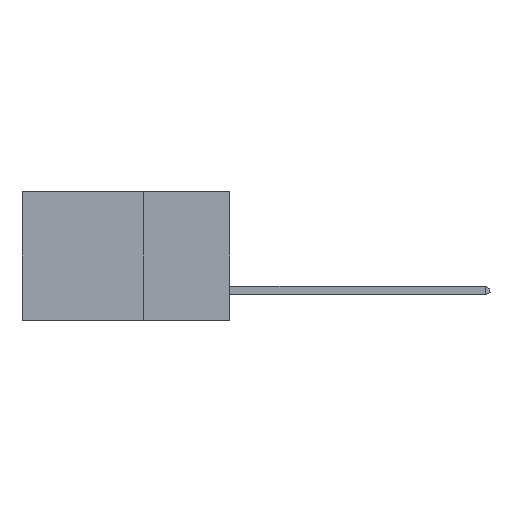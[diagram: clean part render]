
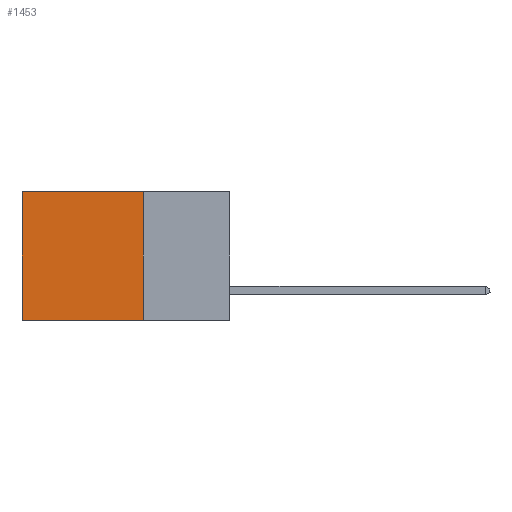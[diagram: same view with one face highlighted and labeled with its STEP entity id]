
A CAD part, left-side view. The second image highlights one B-rep face of the part: STEP entity #1453.
In plain terms, the highlighted planar face has unit normal (-1, 0, 0).
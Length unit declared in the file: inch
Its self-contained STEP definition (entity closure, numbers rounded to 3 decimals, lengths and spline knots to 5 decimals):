
#591 = VERTEX_POINT ( 'NONE', #19879 ) ;
#1293 = EDGE_LOOP ( 'NONE', ( #11337, #5749, #17650, #3230 ) ) ;
#1453 = ADVANCED_FACE ( 'NONE', ( #4125 ), #7468, .F. ) ;
#1702 = VECTOR ( 'NONE', #20775, 39.37008 ) ;
#2573 = DIRECTION ( 'NONE',  ( 0., 0., -1. ) ) ;
#2679 = CARTESIAN_POINT ( 'NONE',  ( 0.298, 0.6, 0. ) ) ;
#2798 = VECTOR ( 'NONE', #12227, 39.37008 ) ;
#3116 = CARTESIAN_POINT ( 'NONE',  ( 0.298, 0.25, -0.37 ) ) ;
#3230 = ORIENTED_EDGE ( 'NONE', *, *, #4395, .T. ) ;
#3769 = VERTEX_POINT ( 'NONE', #10613 ) ;
#4125 = FACE_OUTER_BOUND ( 'NONE', #1293, .T. ) ;
#4395 = EDGE_CURVE ( 'NONE', #3769, #591, #15009, .T. ) ;
#5201 = EDGE_CURVE ( 'NONE', #591, #13915, #13582, .T. ) ;
#5749 = ORIENTED_EDGE ( 'NONE', *, *, #13955, .F. ) ;
#7468 = PLANE ( 'NONE',  #7604 ) ;
#7575 = VERTEX_POINT ( 'NONE', #3116 ) ;
#7604 = AXIS2_PLACEMENT_3D ( 'NONE', #18909, #10744, #2573 ) ;
#7611 = CARTESIAN_POINT ( 'NONE',  ( 0.298, 0.25, -0.37 ) ) ;
#8381 = LINE ( 'NONE', #7611, #1702 ) ;
#9285 = CARTESIAN_POINT ( 'NONE',  ( 0.298, 0.25, 0. ) ) ;
#9339 = DIRECTION ( 'NONE',  ( 0., 0., -1. ) ) ;
#9612 = CARTESIAN_POINT ( 'NONE',  ( 0.298, 0.25, 0. ) ) ;
#10613 = CARTESIAN_POINT ( 'NONE',  ( 0.298, 0.25, 0. ) ) ;
#10744 = DIRECTION ( 'NONE',  ( 1., 0., 0. ) ) ;
#11337 = ORIENTED_EDGE ( 'NONE', *, *, #5201, .T. ) ;
#11869 = EDGE_CURVE ( 'NONE', #3769, #7575, #14130, .T. ) ;
#12227 = DIRECTION ( 'NONE',  ( 0., 0., -1. ) ) ;
#13582 = LINE ( 'NONE', #2679, #2798 ) ;
#13618 = VECTOR ( 'NONE', #9339, 39.37008 ) ;
#13915 = VERTEX_POINT ( 'NONE', #20843 ) ;
#13955 = EDGE_CURVE ( 'NONE', #7575, #13915, #8381, .T. ) ;
#14130 = LINE ( 'NONE', #9285, #13618 ) ;
#15009 = LINE ( 'NONE', #9612, #18083 ) ;
#17650 = ORIENTED_EDGE ( 'NONE', *, *, #11869, .F. ) ;
#18083 = VECTOR ( 'NONE', #21067, 39.37008 ) ;
#18909 = CARTESIAN_POINT ( 'NONE',  ( 0.298, 0.25, 0. ) ) ;
#19879 = CARTESIAN_POINT ( 'NONE',  ( 0.298, 0.6, 0. ) ) ;
#20775 = DIRECTION ( 'NONE',  ( 0., 1., 0. ) ) ;
#20843 = CARTESIAN_POINT ( 'NONE',  ( 0.298, 0.6, -0.37 ) ) ;
#21067 = DIRECTION ( 'NONE',  ( 0., 1., 0. ) ) ;
